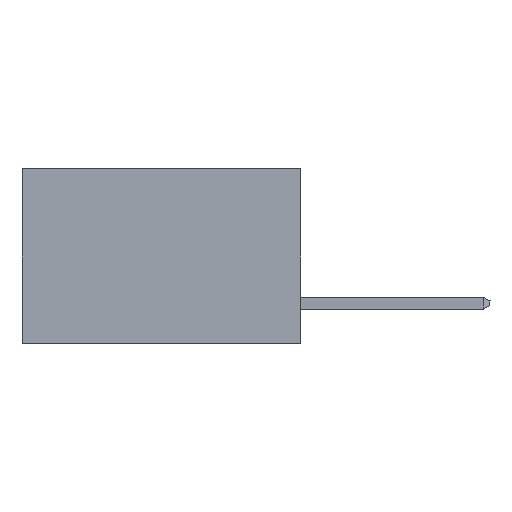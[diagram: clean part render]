
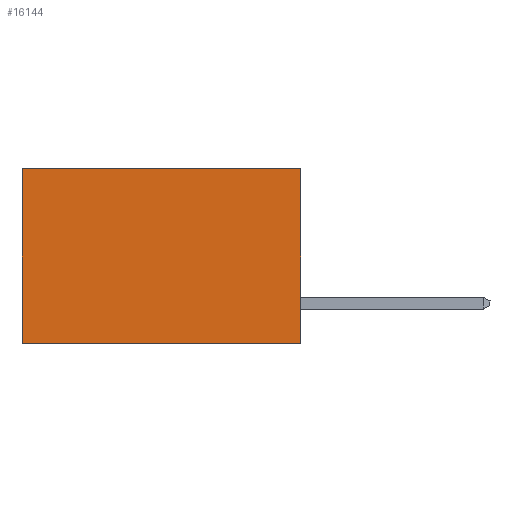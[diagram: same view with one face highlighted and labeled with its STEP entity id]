
A CAD part, left-side view. The second image highlights one B-rep face of the part: STEP entity #16144.
In plain terms, the highlighted planar face has unit normal (-1, 0, 0).
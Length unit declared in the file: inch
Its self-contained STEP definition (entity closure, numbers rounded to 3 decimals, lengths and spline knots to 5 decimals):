
#1227 = VERTEX_POINT ( 'NONE', #6581 ) ;
#1637 = VECTOR ( 'NONE', #24570, 39.37008 ) ;
#1745 = CARTESIAN_POINT ( 'NONE',  ( 0.277, 0., -0.37 ) ) ;
#2272 = LINE ( 'NONE', #24596, #1637 ) ;
#2298 = ORIENTED_EDGE ( 'NONE', *, *, #24017, .T. ) ;
#2323 = ORIENTED_EDGE ( 'NONE', *, *, #6624, .T. ) ;
#2340 = VECTOR ( 'NONE', #11858, 39.37008 ) ;
#2825 = EDGE_CURVE ( 'NONE', #14053, #1227, #22038, .T. ) ;
#3400 = DIRECTION ( 'NONE',  ( 1., 0., 0. ) ) ;
#4199 = ORIENTED_EDGE ( 'NONE', *, *, #2825, .F. ) ;
#6581 = CARTESIAN_POINT ( 'NONE',  ( 0.277, 0., -0.37 ) ) ;
#6624 = EDGE_CURVE ( 'NONE', #14053, #16000, #2272, .T. ) ;
#7945 = FACE_OUTER_BOUND ( 'NONE', #18457, .T. ) ;
#9276 = CARTESIAN_POINT ( 'NONE',  ( 0.277, 0., -0.37 ) ) ;
#9942 = CARTESIAN_POINT ( 'NONE',  ( 0.277, 0.59, -0.37 ) ) ;
#10097 = AXIS2_PLACEMENT_3D ( 'NONE', #9276, #3400, #17069 ) ;
#10727 = VECTOR ( 'NONE', #20355, 39.37008 ) ;
#11346 = VERTEX_POINT ( 'NONE', #9942 ) ;
#11761 = VECTOR ( 'NONE', #20906, 39.37008 ) ;
#11858 = DIRECTION ( 'NONE',  ( 0., 1., 0. ) ) ;
#14053 = VERTEX_POINT ( 'NONE', #14804 ) ;
#14804 = CARTESIAN_POINT ( 'NONE',  ( 0.277, 0., 0. ) ) ;
#15078 = PLANE ( 'NONE',  #10097 ) ;
#15748 = CARTESIAN_POINT ( 'NONE',  ( 0.277, 0., -0.37 ) ) ;
#16000 = VERTEX_POINT ( 'NONE', #20530 ) ;
#16144 = ADVANCED_FACE ( 'NONE', ( #7945 ), #15078, .F. ) ;
#16381 = EDGE_CURVE ( 'NONE', #1227, #11346, #17366, .T. ) ;
#17069 = DIRECTION ( 'NONE',  ( 0., 0., -1. ) ) ;
#17366 = LINE ( 'NONE', #15748, #2340 ) ;
#18457 = EDGE_LOOP ( 'NONE', ( #2298, #18510, #4199, #2323 ) ) ;
#18510 = ORIENTED_EDGE ( 'NONE', *, *, #16381, .F. ) ;
#20355 = DIRECTION ( 'NONE',  ( 0., 0., -1. ) ) ;
#20444 = LINE ( 'NONE', #24202, #10727 ) ;
#20530 = CARTESIAN_POINT ( 'NONE',  ( 0.277, 0.59, 0. ) ) ;
#20906 = DIRECTION ( 'NONE',  ( 0., 0., -1. ) ) ;
#22038 = LINE ( 'NONE', #1745, #11761 ) ;
#24017 = EDGE_CURVE ( 'NONE', #16000, #11346, #20444, .T. ) ;
#24202 = CARTESIAN_POINT ( 'NONE',  ( 0.277, 0.59, -0.37 ) ) ;
#24570 = DIRECTION ( 'NONE',  ( 0., 1., 0. ) ) ;
#24596 = CARTESIAN_POINT ( 'NONE',  ( 0.277, 0., 0. ) ) ;
